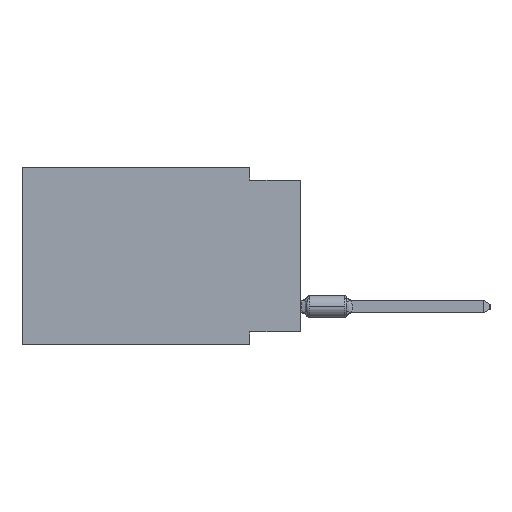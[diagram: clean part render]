
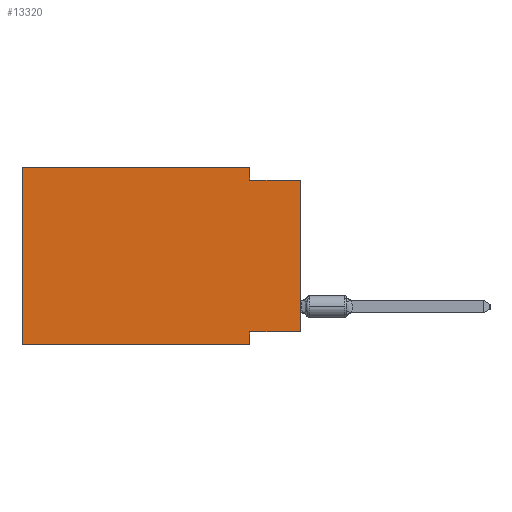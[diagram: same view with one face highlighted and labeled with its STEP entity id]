
A CAD part, left-side view. The second image highlights one B-rep face of the part: STEP entity #13320.
In plain terms, the highlighted planar face has unit normal (-1, 0, 0).
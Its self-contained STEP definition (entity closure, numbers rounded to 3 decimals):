
#1967 = VERTEX_POINT ( 'NONE', #50165 ) ;
#2124 = DIRECTION ( 'NONE',  ( 0., -1., 0. ) ) ;
#2299 = ORIENTED_EDGE ( 'NONE', *, *, #3608, .F. ) ;
#3608 = EDGE_CURVE ( 'NONE', #10622, #1967, #58235, .T. ) ;
#5044 = LINE ( 'NONE', #5641, #44493 ) ;
#5641 = CARTESIAN_POINT ( 'NONE',  ( 0., 13.97, 0. ) ) ;
#7187 = VERTEX_POINT ( 'NONE', #23033 ) ;
#10375 = PLANE ( 'NONE',  #25386 ) ;
#10622 = VERTEX_POINT ( 'NONE', #56022 ) ;
#10960 = DIRECTION ( 'NONE',  ( 1., 0., 0. ) ) ;
#11502 = CARTESIAN_POINT ( 'NONE',  ( 0., 0., -0.635 ) ) ;
#11980 = CARTESIAN_POINT ( 'NONE',  ( 0., 0., -0.635 ) ) ;
#12403 = CARTESIAN_POINT ( 'NONE',  ( 0., 13.97, 0. ) ) ;
#13320 = ADVANCED_FACE ( 'NONE', ( #23993 ), #10375, .F. ) ;
#13592 = ORIENTED_EDGE ( 'NONE', *, *, #57186, .T. ) ;
#15277 = VECTOR ( 'NONE', #34620, 1000. ) ;
#15846 = ORIENTED_EDGE ( 'NONE', *, *, #50579, .F. ) ;
#16106 = VECTOR ( 'NONE', #2124, 1000. ) ;
#17608 = EDGE_CURVE ( 'NONE', #27820, #33698, #22712, .T. ) ;
#19219 = EDGE_CURVE ( 'NONE', #38409, #41818, #29786, .T. ) ;
#20582 = LINE ( 'NONE', #11502, #16106 ) ;
#21266 = DIRECTION ( 'NONE',  ( 0., -1., 0. ) ) ;
#21549 = LINE ( 'NONE', #40004, #49487 ) ;
#22712 = LINE ( 'NONE', #42082, #47019 ) ;
#23033 = CARTESIAN_POINT ( 'NONE',  ( 0., 2.54, -0.635 ) ) ;
#23993 = FACE_OUTER_BOUND ( 'NONE', #43096, .T. ) ;
#24872 = CARTESIAN_POINT ( 'NONE',  ( 0., 2.54, 0. ) ) ;
#25386 = AXIS2_PLACEMENT_3D ( 'NONE', #28844, #10960, #29724 ) ;
#27820 = VERTEX_POINT ( 'NONE', #54887 ) ;
#28401 = EDGE_CURVE ( 'NONE', #7187, #33698, #20582, .T. ) ;
#28844 = CARTESIAN_POINT ( 'NONE',  ( 0., 13.97, 0. ) ) ;
#29724 = DIRECTION ( 'NONE',  ( 0., 0., -1. ) ) ;
#29786 = LINE ( 'NONE', #58209, #31349 ) ;
#30607 = VECTOR ( 'NONE', #49175, 1000. ) ;
#31349 = VECTOR ( 'NONE', #40346, 1000. ) ;
#33006 = ORIENTED_EDGE ( 'NONE', *, *, #46258, .F. ) ;
#33698 = VERTEX_POINT ( 'NONE', #11980 ) ;
#34044 = EDGE_CURVE ( 'NONE', #41818, #7187, #51613, .T. ) ;
#34620 = DIRECTION ( 'NONE',  ( 0., 1., 0. ) ) ;
#36621 = ORIENTED_EDGE ( 'NONE', *, *, #19219, .F. ) ;
#37205 = CARTESIAN_POINT ( 'NONE',  ( 0., 13.97, -8.89 ) ) ;
#37558 = DIRECTION ( 'NONE',  ( 0., 0., 1. ) ) ;
#38409 = VERTEX_POINT ( 'NONE', #12403 ) ;
#40004 = CARTESIAN_POINT ( 'NONE',  ( 0., 13.97, -8.89 ) ) ;
#40346 = DIRECTION ( 'NONE',  ( 0., -1., 0. ) ) ;
#41818 = VERTEX_POINT ( 'NONE', #50763 ) ;
#42082 = CARTESIAN_POINT ( 'NONE',  ( 0., 0., 0. ) ) ;
#43096 = EDGE_LOOP ( 'NONE', ( #47082, #55561, #51663, #36621, #15846, #13592, #2299, #33006 ) ) ;
#43337 = DIRECTION ( 'NONE',  ( 0., 0., -1. ) ) ;
#43991 = CARTESIAN_POINT ( 'NONE',  ( 0., 0., -8.255 ) ) ;
#44493 = VECTOR ( 'NONE', #56779, 1000. ) ;
#46258 = EDGE_CURVE ( 'NONE', #27820, #10622, #58493, .T. ) ;
#47019 = VECTOR ( 'NONE', #37558, 1000. ) ;
#47082 = ORIENTED_EDGE ( 'NONE', *, *, #17608, .T. ) ;
#49175 = DIRECTION ( 'NONE',  ( 0., 0., -1. ) ) ;
#49487 = VECTOR ( 'NONE', #21266, 1000. ) ;
#50113 = VERTEX_POINT ( 'NONE', #37205 ) ;
#50165 = CARTESIAN_POINT ( 'NONE',  ( 0., 2.54, -8.89 ) ) ;
#50579 = EDGE_CURVE ( 'NONE', #50113, #38409, #5044, .T. ) ;
#50763 = CARTESIAN_POINT ( 'NONE',  ( 0., 2.54, 0. ) ) ;
#51613 = LINE ( 'NONE', #24872, #59659 ) ;
#51663 = ORIENTED_EDGE ( 'NONE', *, *, #34044, .F. ) ;
#54887 = CARTESIAN_POINT ( 'NONE',  ( 0., 0., -8.255 ) ) ;
#55561 = ORIENTED_EDGE ( 'NONE', *, *, #28401, .F. ) ;
#56022 = CARTESIAN_POINT ( 'NONE',  ( 0., 2.54, -8.255 ) ) ;
#56779 = DIRECTION ( 'NONE',  ( 0., 0., 1. ) ) ;
#57186 = EDGE_CURVE ( 'NONE', #50113, #1967, #21549, .T. ) ;
#58209 = CARTESIAN_POINT ( 'NONE',  ( 0., 13.97, 0. ) ) ;
#58235 = LINE ( 'NONE', #58535, #30607 ) ;
#58493 = LINE ( 'NONE', #43991, #15277 ) ;
#58535 = CARTESIAN_POINT ( 'NONE',  ( 0., 2.54, -8.89 ) ) ;
#59659 = VECTOR ( 'NONE', #43337, 1000. ) ;
